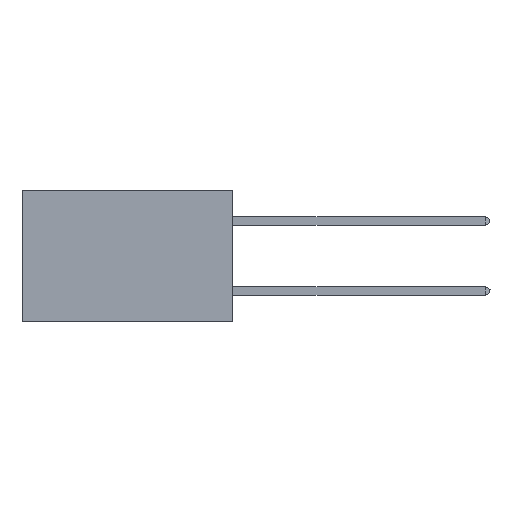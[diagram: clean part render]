
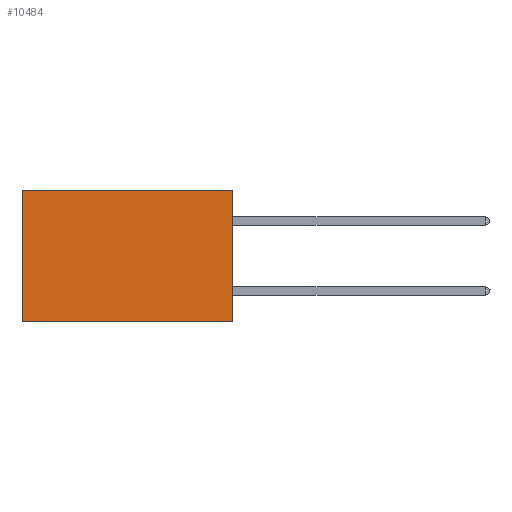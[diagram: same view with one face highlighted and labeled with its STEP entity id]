
A CAD part, left-side view. The second image highlights one B-rep face of the part: STEP entity #10484.
In plain terms, the highlighted planar face has unit normal (-1, 0, 0).
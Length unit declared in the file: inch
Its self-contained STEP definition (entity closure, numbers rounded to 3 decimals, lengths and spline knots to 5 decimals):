
#474 = ORIENTED_EDGE ( 'NONE', *, *, #2179, .F. ) ;
#519 = VERTEX_POINT ( 'NONE', #9346 ) ;
#581 = DIRECTION ( 'NONE',  ( 1., 0., 0. ) ) ;
#615 = VECTOR ( 'NONE', #9719, 39.37008 ) ;
#1181 = VECTOR ( 'NONE', #10310, 39.37008 ) ;
#1504 = EDGE_CURVE ( 'NONE', #13609, #5374, #15333, .T. ) ;
#1832 = DIRECTION ( 'NONE',  ( 0., 0., -1. ) ) ;
#1944 = CARTESIAN_POINT ( 'NONE',  ( 0.2875, 0., -0.375 ) ) ;
#2179 = EDGE_CURVE ( 'NONE', #5374, #14351, #5984, .T. ) ;
#3217 = ORIENTED_EDGE ( 'NONE', *, *, #1504, .F. ) ;
#3262 = LINE ( 'NONE', #5550, #1181 ) ;
#3322 = CARTESIAN_POINT ( 'NONE',  ( 0.2875, 0., -0.375 ) ) ;
#3374 = EDGE_LOOP ( 'NONE', ( #11030, #474, #3217, #12606 ) ) ;
#3465 = FACE_OUTER_BOUND ( 'NONE', #3374, .T. ) ;
#4207 = LINE ( 'NONE', #14276, #615 ) ;
#5353 = CARTESIAN_POINT ( 'NONE',  ( 0.2875, 0., -0.375 ) ) ;
#5374 = VERTEX_POINT ( 'NONE', #9064 ) ;
#5465 = VECTOR ( 'NONE', #5815, 39.37008 ) ;
#5550 = CARTESIAN_POINT ( 'NONE',  ( 0.2875, 0., 0. ) ) ;
#5815 = DIRECTION ( 'NONE',  ( 0., 1., 0. ) ) ;
#5984 = LINE ( 'NONE', #3322, #5465 ) ;
#7063 = EDGE_CURVE ( 'NONE', #519, #14351, #4207, .T. ) ;
#7544 = CARTESIAN_POINT ( 'NONE',  ( 0.2875, 0., 0. ) ) ;
#8927 = DIRECTION ( 'NONE',  ( 0., 0., -1. ) ) ;
#9064 = CARTESIAN_POINT ( 'NONE',  ( 0.2875, 0., -0.375 ) ) ;
#9346 = CARTESIAN_POINT ( 'NONE',  ( 0.2875, 0.6, 0. ) ) ;
#9719 = DIRECTION ( 'NONE',  ( 0., 0., -1. ) ) ;
#10310 = DIRECTION ( 'NONE',  ( 0., 1., 0. ) ) ;
#10344 = CARTESIAN_POINT ( 'NONE',  ( 0.2875, 0.6, -0.375 ) ) ;
#10484 = ADVANCED_FACE ( 'NONE', ( #3465 ), #14840, .F. ) ;
#11030 = ORIENTED_EDGE ( 'NONE', *, *, #7063, .T. ) ;
#11144 = EDGE_CURVE ( 'NONE', #13609, #519, #3262, .T. ) ;
#11219 = VECTOR ( 'NONE', #1832, 39.37008 ) ;
#12606 = ORIENTED_EDGE ( 'NONE', *, *, #11144, .T. ) ;
#13609 = VERTEX_POINT ( 'NONE', #7544 ) ;
#13974 = AXIS2_PLACEMENT_3D ( 'NONE', #5353, #581, #8927 ) ;
#14276 = CARTESIAN_POINT ( 'NONE',  ( 0.2875, 0.6, -0.375 ) ) ;
#14351 = VERTEX_POINT ( 'NONE', #10344 ) ;
#14840 = PLANE ( 'NONE',  #13974 ) ;
#15333 = LINE ( 'NONE', #1944, #11219 ) ;
